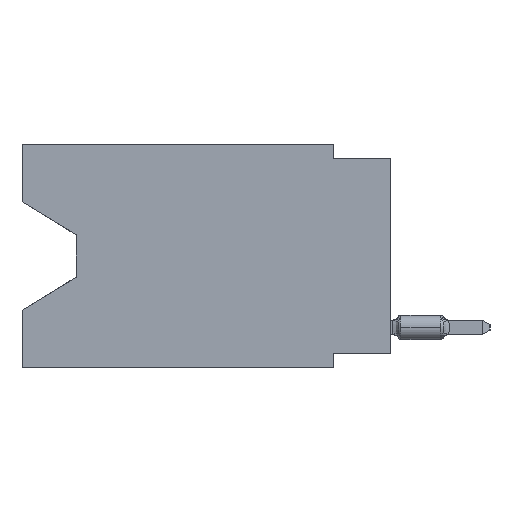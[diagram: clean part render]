
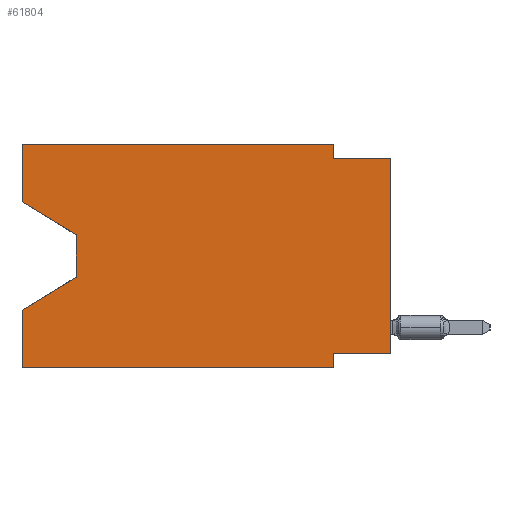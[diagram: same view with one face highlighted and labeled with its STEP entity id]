
A CAD part, left-side view. The second image highlights one B-rep face of the part: STEP entity #61804.
In plain terms, the highlighted planar face has unit normal (-1, 0, 0).
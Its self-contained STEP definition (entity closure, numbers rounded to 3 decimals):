
#198 = CARTESIAN_POINT ( 'NONE',  ( 0., 16.383, 0. ) ) ;
#1305 = CARTESIAN_POINT ( 'NONE',  ( 0., 16.383, 0. ) ) ;
#2285 = VERTEX_POINT ( 'NONE', #66173 ) ;
#3403 = CARTESIAN_POINT ( 'NONE',  ( 0., 2.54, -0.635 ) ) ;
#4105 = ORIENTED_EDGE ( 'NONE', *, *, #50443, .F. ) ;
#4503 = DIRECTION ( 'NONE',  ( 0., 0., 1. ) ) ;
#5066 = LINE ( 'NONE', #70715, #79035 ) ;
#5157 = CARTESIAN_POINT ( 'NONE',  ( 0., 0., 0. ) ) ;
#5742 = LINE ( 'NONE', #19551, #58999 ) ;
#6334 = EDGE_CURVE ( 'NONE', #22623, #18128, #44881, .T. ) ;
#6862 = VERTEX_POINT ( 'NONE', #70284 ) ;
#8354 = CARTESIAN_POINT ( 'NONE',  ( 0., 0., -9.271 ) ) ;
#9521 = ORIENTED_EDGE ( 'NONE', *, *, #36000, .T. ) ;
#11390 = LINE ( 'NONE', #30821, #48161 ) ;
#12897 = VECTOR ( 'NONE', #18390, 1000. ) ;
#14029 = LINE ( 'NONE', #42067, #52568 ) ;
#14345 = CARTESIAN_POINT ( 'NONE',  ( 0., 0., -0.635 ) ) ;
#15055 = VERTEX_POINT ( 'NONE', #198 ) ;
#15427 = DIRECTION ( 'NONE',  ( 0., 0., -1. ) ) ;
#15616 = LINE ( 'NONE', #54500, #51030 ) ;
#17591 = DIRECTION ( 'NONE',  ( 0., 0., -1. ) ) ;
#18128 = VERTEX_POINT ( 'NONE', #14345 ) ;
#18390 = DIRECTION ( 'NONE',  ( 0., -1., 0. ) ) ;
#18589 = EDGE_CURVE ( 'NONE', #29349, #39885, #79409, .T. ) ;
#18620 = CARTESIAN_POINT ( 'NONE',  ( 0., 16.383, -9.906 ) ) ;
#19020 = PLANE ( 'NONE',  #78289 ) ;
#19279 = VECTOR ( 'NONE', #34961, 1000. ) ;
#19551 = CARTESIAN_POINT ( 'NONE',  ( 0., 13.97, -4.013 ) ) ;
#19564 = VERTEX_POINT ( 'NONE', #70901 ) ;
#19881 = DIRECTION ( 'NONE',  ( 1., 0., 0. ) ) ;
#20631 = DIRECTION ( 'NONE',  ( 0., 0.855, -0.519 ) ) ;
#21241 = DIRECTION ( 'NONE',  ( 0., 0., 1. ) ) ;
#21400 = ORIENTED_EDGE ( 'NONE', *, *, #83841, .F. ) ;
#22029 = EDGE_CURVE ( 'NONE', #19564, #2285, #5066, .T. ) ;
#22329 = CARTESIAN_POINT ( 'NONE',  ( 0., 2.54, 0. ) ) ;
#22623 = VERTEX_POINT ( 'NONE', #8354 ) ;
#24575 = CARTESIAN_POINT ( 'NONE',  ( 0., 13.97, -4.013 ) ) ;
#26044 = CARTESIAN_POINT ( 'NONE',  ( 0., 0., -0.635 ) ) ;
#27888 = EDGE_CURVE ( 'NONE', #69875, #29349, #5742, .T. ) ;
#29333 = LINE ( 'NONE', #62179, #19279 ) ;
#29349 = VERTEX_POINT ( 'NONE', #64297 ) ;
#30821 = CARTESIAN_POINT ( 'NONE',  ( 0., 16.383, 0. ) ) ;
#32412 = VECTOR ( 'NONE', #40582, 1000. ) ;
#34562 = ORIENTED_EDGE ( 'NONE', *, *, #42250, .F. ) ;
#34714 = EDGE_CURVE ( 'NONE', #76682, #52296, #62075, .T. ) ;
#34961 = DIRECTION ( 'NONE',  ( 0., 1., 0. ) ) ;
#36000 = EDGE_CURVE ( 'NONE', #54992, #2285, #63761, .T. ) ;
#37265 = ORIENTED_EDGE ( 'NONE', *, *, #45297, .T. ) ;
#39885 = VERTEX_POINT ( 'NONE', #50120 ) ;
#40582 = DIRECTION ( 'NONE',  ( 0., -1., 0. ) ) ;
#42067 = CARTESIAN_POINT ( 'NONE',  ( 0., 16.383, -2.546 ) ) ;
#42250 = EDGE_CURVE ( 'NONE', #54992, #39885, #15616, .T. ) ;
#43882 = CARTESIAN_POINT ( 'NONE',  ( 0., 16.383, -9.906 ) ) ;
#44881 = LINE ( 'NONE', #5157, #53409 ) ;
#45239 = ORIENTED_EDGE ( 'NONE', *, *, #18589, .T. ) ;
#45297 = EDGE_CURVE ( 'NONE', #6862, #69875, #14029, .T. ) ;
#46207 = CARTESIAN_POINT ( 'NONE',  ( 0., 16.383, 0. ) ) ;
#46842 = EDGE_CURVE ( 'NONE', #52296, #18128, #65812, .T. ) ;
#47256 = DIRECTION ( 'NONE',  ( 0., -0.855, -0.519 ) ) ;
#48161 = VECTOR ( 'NONE', #4503, 1000. ) ;
#48605 = ORIENTED_EDGE ( 'NONE', *, *, #83187, .F. ) ;
#50120 = CARTESIAN_POINT ( 'NONE',  ( 0., 16.383, -7.36 ) ) ;
#50443 = EDGE_CURVE ( 'NONE', #15055, #76682, #72594, .T. ) ;
#51030 = VECTOR ( 'NONE', #21241, 1000. ) ;
#52296 = VERTEX_POINT ( 'NONE', #3403 ) ;
#52568 = VECTOR ( 'NONE', #47256, 1000. ) ;
#53409 = VECTOR ( 'NONE', #78156, 1000. ) ;
#54500 = CARTESIAN_POINT ( 'NONE',  ( 0., 16.383, 0. ) ) ;
#54604 = ORIENTED_EDGE ( 'NONE', *, *, #6334, .T. ) ;
#54934 = CARTESIAN_POINT ( 'NONE',  ( 0., 2.54, 0. ) ) ;
#54992 = VERTEX_POINT ( 'NONE', #18620 ) ;
#58999 = VECTOR ( 'NONE', #72252, 1000. ) ;
#59187 = DIRECTION ( 'NONE',  ( 0., 0., -1. ) ) ;
#61767 = ORIENTED_EDGE ( 'NONE', *, *, #27888, .T. ) ;
#61804 = ADVANCED_FACE ( 'NONE', ( #85090 ), #19020, .F. ) ;
#62075 = LINE ( 'NONE', #22329, #76241 ) ;
#62179 = CARTESIAN_POINT ( 'NONE',  ( 0., 0., -9.271 ) ) ;
#63761 = LINE ( 'NONE', #43882, #12897 ) ;
#64297 = CARTESIAN_POINT ( 'NONE',  ( 0., 13.97, -5.893 ) ) ;
#65812 = LINE ( 'NONE', #26044, #74924 ) ;
#66173 = CARTESIAN_POINT ( 'NONE',  ( 0., 2.54, -9.906 ) ) ;
#66484 = ORIENTED_EDGE ( 'NONE', *, *, #46842, .F. ) ;
#69875 = VERTEX_POINT ( 'NONE', #24575 ) ;
#70284 = CARTESIAN_POINT ( 'NONE',  ( 0., 16.383, -2.546 ) ) ;
#70715 = CARTESIAN_POINT ( 'NONE',  ( 0., 2.54, -9.906 ) ) ;
#70809 = ORIENTED_EDGE ( 'NONE', *, *, #22029, .F. ) ;
#70901 = CARTESIAN_POINT ( 'NONE',  ( 0., 2.54, -9.271 ) ) ;
#72252 = DIRECTION ( 'NONE',  ( 0., 0., -1. ) ) ;
#72594 = LINE ( 'NONE', #1305, #32412 ) ;
#74924 = VECTOR ( 'NONE', #78774, 1000. ) ;
#76241 = VECTOR ( 'NONE', #15427, 1000. ) ;
#76682 = VERTEX_POINT ( 'NONE', #54934 ) ;
#78156 = DIRECTION ( 'NONE',  ( 0., 0., 1. ) ) ;
#78289 = AXIS2_PLACEMENT_3D ( 'NONE', #46207, #19881, #59187 ) ;
#78774 = DIRECTION ( 'NONE',  ( 0., -1., 0. ) ) ;
#79035 = VECTOR ( 'NONE', #17591, 1000. ) ;
#79313 = ORIENTED_EDGE ( 'NONE', *, *, #34714, .F. ) ;
#79409 = LINE ( 'NONE', #79827, #83018 ) ;
#79827 = CARTESIAN_POINT ( 'NONE',  ( 0., 13.97, -5.893 ) ) ;
#79962 = EDGE_LOOP ( 'NONE', ( #37265, #61767, #45239, #34562, #9521, #70809, #21400, #54604, #66484, #79313, #4105, #48605 ) ) ;
#83018 = VECTOR ( 'NONE', #20631, 1000. ) ;
#83187 = EDGE_CURVE ( 'NONE', #6862, #15055, #11390, .T. ) ;
#83841 = EDGE_CURVE ( 'NONE', #22623, #19564, #29333, .T. ) ;
#85090 = FACE_OUTER_BOUND ( 'NONE', #79962, .T. ) ;
